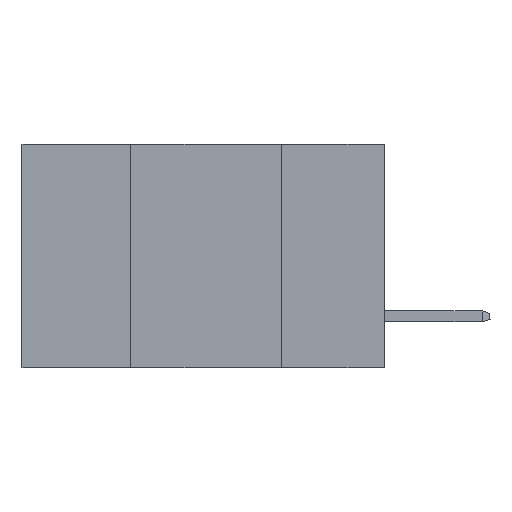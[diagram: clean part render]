
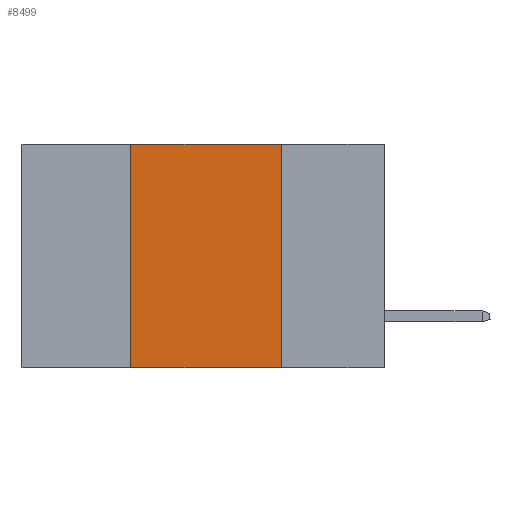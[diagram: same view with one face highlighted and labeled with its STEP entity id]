
A CAD part, left-side view. The second image highlights one B-rep face of the part: STEP entity #8499.
In plain terms, the highlighted planar face has unit normal (-1, 0, 0).
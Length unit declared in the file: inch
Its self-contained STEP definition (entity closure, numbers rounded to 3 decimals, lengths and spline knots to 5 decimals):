
#95 = ORIENTED_EDGE ( 'NONE', *, *, #6393, .F. ) ;
#118 = LINE ( 'NONE', #2930, #2580 ) ;
#148 = ORIENTED_EDGE ( 'NONE', *, *, #6405, .T. ) ;
#728 = VERTEX_POINT ( 'NONE', #5170 ) ;
#839 = ORIENTED_EDGE ( 'NONE', *, *, #4407, .F. ) ;
#1069 = ORIENTED_EDGE ( 'NONE', *, *, #6360, .F. ) ;
#1447 = VECTOR ( 'NONE', #2970, 39.37008 ) ;
#1613 = AXIS2_PLACEMENT_3D ( 'NONE', #6312, #9098, #4880 ) ;
#1739 = LINE ( 'NONE', #6702, #7419 ) ;
#2580 = VECTOR ( 'NONE', #7396, 39.37008 ) ;
#2930 = CARTESIAN_POINT ( 'NONE',  ( 0., 0.17, 0. ) ) ;
#2970 = DIRECTION ( 'NONE',  ( 0., 0., 1. ) ) ;
#3141 = LINE ( 'NONE', #7978, #3383 ) ;
#3383 = VECTOR ( 'NONE', #7995, 39.37008 ) ;
#3720 = FACE_OUTER_BOUND ( 'NONE', #9045, .T. ) ;
#3848 = VERTEX_POINT ( 'NONE', #7552 ) ;
#4113 = PLANE ( 'NONE',  #1613 ) ;
#4407 = EDGE_CURVE ( 'NONE', #728, #9515, #3141, .T. ) ;
#4525 = DIRECTION ( 'NONE',  ( 0., -1., 0. ) ) ;
#4880 = DIRECTION ( 'NONE',  ( 0., 0., -1. ) ) ;
#5170 = CARTESIAN_POINT ( 'NONE',  ( 0., 0.42, 0. ) ) ;
#5268 = CARTESIAN_POINT ( 'NONE',  ( 0., 0.42, 0. ) ) ;
#5473 = CARTESIAN_POINT ( 'NONE',  ( 0., 0.17, 0. ) ) ;
#5770 = LINE ( 'NONE', #5268, #1447 ) ;
#6312 = CARTESIAN_POINT ( 'NONE',  ( 0., 0.6, 0. ) ) ;
#6360 = EDGE_CURVE ( 'NONE', #9515, #6777, #118, .T. ) ;
#6393 = EDGE_CURVE ( 'NONE', #3848, #728, #5770, .T. ) ;
#6405 = EDGE_CURVE ( 'NONE', #3848, #6777, #1739, .T. ) ;
#6702 = CARTESIAN_POINT ( 'NONE',  ( 0., 0.6, -0.37 ) ) ;
#6777 = VERTEX_POINT ( 'NONE', #9715 ) ;
#7396 = DIRECTION ( 'NONE',  ( 0., 0., -1. ) ) ;
#7419 = VECTOR ( 'NONE', #4525, 39.37008 ) ;
#7552 = CARTESIAN_POINT ( 'NONE',  ( 0., 0.42, -0.37 ) ) ;
#7978 = CARTESIAN_POINT ( 'NONE',  ( 0., 0.6, 0. ) ) ;
#7995 = DIRECTION ( 'NONE',  ( 0., -1., 0. ) ) ;
#8499 = ADVANCED_FACE ( 'NONE', ( #3720 ), #4113, .F. ) ;
#9045 = EDGE_LOOP ( 'NONE', ( #1069, #839, #95, #148 ) ) ;
#9098 = DIRECTION ( 'NONE',  ( 1., 0., 0. ) ) ;
#9515 = VERTEX_POINT ( 'NONE', #5473 ) ;
#9715 = CARTESIAN_POINT ( 'NONE',  ( 0., 0.17, -0.37 ) ) ;
